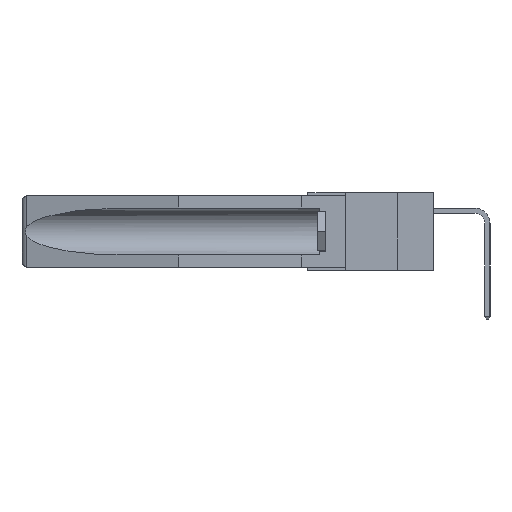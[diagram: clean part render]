
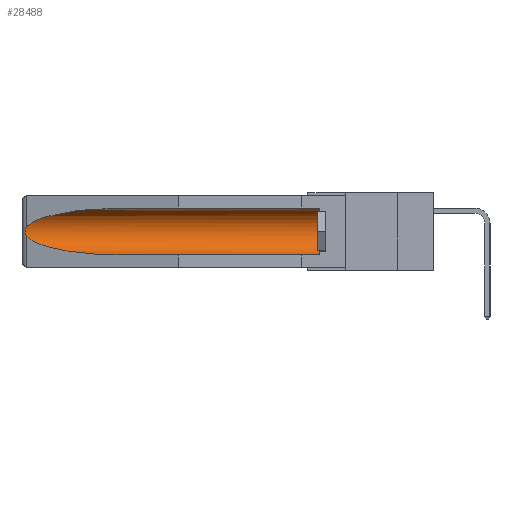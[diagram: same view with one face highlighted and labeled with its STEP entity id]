
A CAD part, left-side view. The second image highlights one B-rep face of the part: STEP entity #28488.
In plain terms, the highlighted cylindrical face has radius 2.857 mm (diameter 5.715 mm), a partial arc.
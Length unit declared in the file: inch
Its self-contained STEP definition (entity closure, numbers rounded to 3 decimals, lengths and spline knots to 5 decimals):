
#216 = VECTOR ( 'NONE', #25947, 39.37008 ) ;
#224 = CARTESIAN_POINT ( 'NONE',  ( 0.25451, 1.48313, -0.24835 ) ) ;
#2018 = DIRECTION ( 'NONE',  ( 0., -1., 0. ) ) ;
#2349 = CARTESIAN_POINT ( 'NONE',  ( 0.25451, 1.48313, -0.09465 ) ) ;
#2932 = AXIS2_PLACEMENT_3D ( 'NONE', #13308, #2018, #16252 ) ;
#3441 = CARTESIAN_POINT ( 'NONE',  ( 0.26655, 1.53094, -0.18657 ) ) ;
#4159 = EDGE_CURVE ( 'NONE', #14716, #19858, #8380, .T. ) ;
#4811 = ORIENTED_EDGE ( 'NONE', *, *, #28332, .F. ) ;
#5471 = CARTESIAN_POINT ( 'NONE',  ( 0.26654, 1.53092, -0.15636 ) ) ;
#5643 = EDGE_CURVE ( 'NONE', #9931, #14716, #16849, .T. ) ;
#5674 = CARTESIAN_POINT ( 'NONE',  ( 0.2675, 1.53308, -0.16763 ) ) ;
#6891 = VERTEX_POINT ( 'NONE', #25175 ) ;
#7201 = CARTESIAN_POINT ( 'NONE',  ( 0.155, -0.30754, -0.1715 ) ) ;
#7723 = CARTESIAN_POINT ( 'NONE',  ( 0.2673, 1.5327, -0.16383 ) ) ;
#7816 = CARTESIAN_POINT ( 'NONE',  ( 0.26537, 1.52718, -0.14972 ) ) ;
#7873 = CARTESIAN_POINT ( 'NONE',  ( 0.155, 0.126, -0.059 ) ) ;
#8083 = CARTESIAN_POINT ( 'NONE',  ( 0.2673, 1.53269, -0.17917 ) ) ;
#8380 =( BOUNDED_CURVE ( )  B_SPLINE_CURVE ( 3, ( #8941, #15690, #2349, #28912 ),
 .UNSPECIFIED., .F., .F. ) 
 B_SPLINE_CURVE_WITH_KNOTS ( ( 4, 4 ),
 ( 4.71239, 6.08839 ),
 .UNSPECIFIED. ) 
 CURVE ( )  GEOMETRIC_REPRESENTATION_ITEM ( )  RATIONAL_B_SPLINE_CURVE ( ( 1., 0.848, 0.848, 1. ) ) 
 REPRESENTATION_ITEM ( '' )  );
#8756 = B_SPLINE_CURVE_WITH_KNOTS ( 'NONE', 3,
 ( #7816, #23544, #5471, #7723, #5674, #21212, #8083, #3441, #21123, #19145 ),
 .UNSPECIFIED., .F., .F.,
 ( 4, 2, 2, 2, 4 ),
 ( 0., 0.00029, 0.00058, 0.00087, 0.00117 ),
 .UNSPECIFIED. ) ;
#8941 = CARTESIAN_POINT ( 'NONE',  ( 0.155, 1.07973, -0.059 ) ) ;
#9931 = VERTEX_POINT ( 'NONE', #7873 ) ;
#10860 = EDGE_CURVE ( 'NONE', #25418, #6891, #14335, .T. ) ;
#10875 = CARTESIAN_POINT ( 'NONE',  ( 0.26537, 1.52718, -0.14972 ) ) ;
#11260 = CARTESIAN_POINT ( 'NONE',  ( 0.155, 1.07973, -0.284 ) ) ;
#12632 = DIRECTION ( 'NONE',  ( 0., 1., 0. ) ) ;
#13182 = ORIENTED_EDGE ( 'NONE', *, *, #5643, .T. ) ;
#13308 = CARTESIAN_POINT ( 'NONE',  ( 0.155, 0.126, -0.1715 ) ) ;
#14031 = ORIENTED_EDGE ( 'NONE', *, *, #10860, .T. ) ;
#14138 = VERTEX_POINT ( 'NONE', #15284 ) ;
#14150 = DIRECTION ( 'NONE',  ( 0., 1., 0. ) ) ;
#14335 =( BOUNDED_CURVE ( )  B_SPLINE_CURVE ( 3, ( #20373, #224, #27017, #11260 ),
 .UNSPECIFIED., .F., .F. ) 
 B_SPLINE_CURVE_WITH_KNOTS ( ( 4, 4 ),
 ( 0.1948, 1.5708 ),
 .UNSPECIFIED. ) 
 CURVE ( )  GEOMETRIC_REPRESENTATION_ITEM ( )  RATIONAL_B_SPLINE_CURVE ( ( 1., 0.848, 0.848, 1. ) ) 
 REPRESENTATION_ITEM ( '' )  );
#14716 = VERTEX_POINT ( 'NONE', #16994 ) ;
#14894 = CARTESIAN_POINT ( 'NONE',  ( 0.155, -0.30754, -0.284 ) ) ;
#15092 = CARTESIAN_POINT ( 'NONE',  ( 0.155, -0.30754, -0.059 ) ) ;
#15284 = CARTESIAN_POINT ( 'NONE',  ( 0.155, 0.126, -0.284 ) ) ;
#15690 = CARTESIAN_POINT ( 'NONE',  ( 0.21114, 1.30732, -0.059 ) ) ;
#16252 = DIRECTION ( 'NONE',  ( 0., 0., 1. ) ) ;
#16849 = LINE ( 'NONE', #15092, #28750 ) ;
#16994 = CARTESIAN_POINT ( 'NONE',  ( 0.155, 1.07973, -0.059 ) ) ;
#18069 = ORIENTED_EDGE ( 'NONE', *, *, #4159, .T. ) ;
#18612 = ORIENTED_EDGE ( 'NONE', *, *, #19115, .T. ) ;
#18630 = CARTESIAN_POINT ( 'NONE',  ( 0.26537, 1.52718, -0.19328 ) ) ;
#19115 = EDGE_CURVE ( 'NONE', #14138, #9931, #21819, .T. ) ;
#19145 = CARTESIAN_POINT ( 'NONE',  ( 0.26537, 1.52718, -0.19328 ) ) ;
#19496 = FACE_OUTER_BOUND ( 'NONE', #26767, .T. ) ;
#19858 = VERTEX_POINT ( 'NONE', #10875 ) ;
#20373 = CARTESIAN_POINT ( 'NONE',  ( 0.26537, 1.52718, -0.19328 ) ) ;
#21123 = CARTESIAN_POINT ( 'NONE',  ( 0.26597, 1.5296, -0.19026 ) ) ;
#21212 = CARTESIAN_POINT ( 'NONE',  ( 0.2675, 1.53308, -0.17534 ) ) ;
#21819 = CIRCLE ( 'NONE', #2932, 0.1125 ) ;
#23417 = ORIENTED_EDGE ( 'NONE', *, *, #24361, .T. ) ;
#23544 = CARTESIAN_POINT ( 'NONE',  ( 0.26597, 1.52961, -0.15275 ) ) ;
#24005 = AXIS2_PLACEMENT_3D ( 'NONE', #7201, #14150, #27633 ) ;
#24048 = CYLINDRICAL_SURFACE ( 'NONE', #24005, 0.1125 ) ;
#24361 = EDGE_CURVE ( 'NONE', #19858, #25418, #8756, .T. ) ;
#25175 = CARTESIAN_POINT ( 'NONE',  ( 0.155, 1.07973, -0.284 ) ) ;
#25418 = VERTEX_POINT ( 'NONE', #18630 ) ;
#25947 = DIRECTION ( 'NONE',  ( 0., 1., 0. ) ) ;
#26767 = EDGE_LOOP ( 'NONE', ( #18069, #23417, #14031, #4811, #18612, #13182 ) ) ;
#27017 = CARTESIAN_POINT ( 'NONE',  ( 0.21114, 1.30732, -0.284 ) ) ;
#27633 = DIRECTION ( 'NONE',  ( 0., 0., 1. ) ) ;
#28212 = LINE ( 'NONE', #14894, #216 ) ;
#28332 = EDGE_CURVE ( 'NONE', #14138, #6891, #28212, .T. ) ;
#28488 = ADVANCED_FACE ( 'NONE', ( #19496 ), #24048, .F. ) ;
#28750 = VECTOR ( 'NONE', #12632, 39.37008 ) ;
#28912 = CARTESIAN_POINT ( 'NONE',  ( 0.26537, 1.52718, -0.14972 ) ) ;
